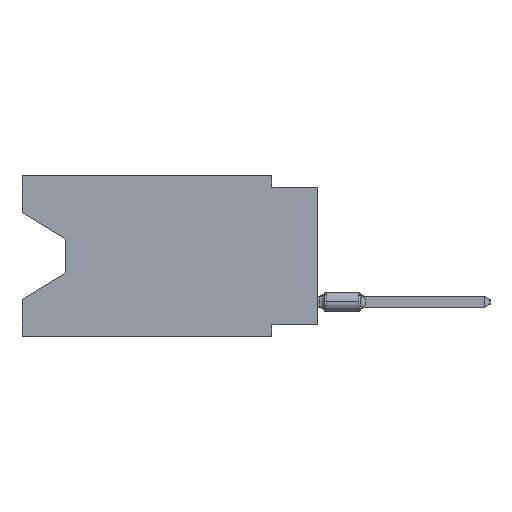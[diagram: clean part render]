
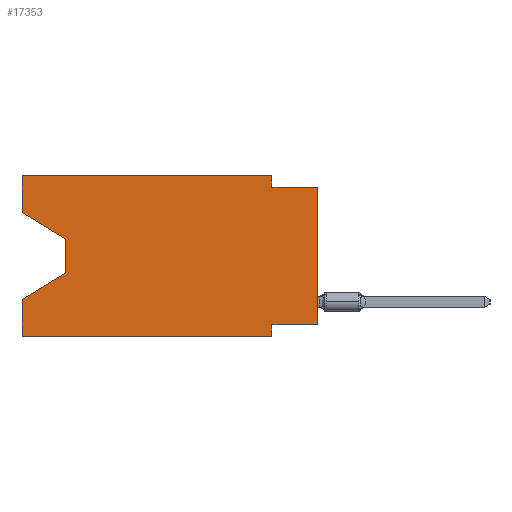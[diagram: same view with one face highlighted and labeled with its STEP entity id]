
A CAD part, left-side view. The second image highlights one B-rep face of the part: STEP entity #17353.
In plain terms, the highlighted planar face has unit normal (-1, 0, 0).
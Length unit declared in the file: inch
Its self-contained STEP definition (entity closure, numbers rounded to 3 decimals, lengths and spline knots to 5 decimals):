
#258 = VECTOR ( 'NONE', #22135, 39.37008 ) ;
#825 = VECTOR ( 'NONE', #10488, 39.37008 ) ;
#1271 = DIRECTION ( 'NONE',  ( 0., 0., -1. ) ) ;
#1423 = EDGE_CURVE ( 'NONE', #21118, #28606, #21655, .T. ) ;
#1750 = VECTOR ( 'NONE', #11403, 39.37008 ) ;
#1928 = ORIENTED_EDGE ( 'NONE', *, *, #2291, .F. ) ;
#2100 = CARTESIAN_POINT ( 'NONE',  ( 0., 0.1, 0. ) ) ;
#2234 = CARTESIAN_POINT ( 'NONE',  ( 0., 0., -0.025 ) ) ;
#2291 = EDGE_CURVE ( 'NONE', #29216, #25674, #48464, .T. ) ;
#3452 = EDGE_CURVE ( 'NONE', #37758, #32745, #3753, .T. ) ;
#3753 = LINE ( 'NONE', #53028, #10088 ) ;
#3994 = ORIENTED_EDGE ( 'NONE', *, *, #34579, .T. ) ;
#4494 = EDGE_CURVE ( 'NONE', #48345, #26114, #19072, .T. ) ;
#5089 = VECTOR ( 'NONE', #7130, 39.37008 ) ;
#6282 = DIRECTION ( 'NONE',  ( 1., 0., 0. ) ) ;
#6395 = EDGE_CURVE ( 'NONE', #21118, #26114, #43600, .T. ) ;
#6995 = CARTESIAN_POINT ( 'NONE',  ( 0., 0.645, 0. ) ) ;
#7130 = DIRECTION ( 'NONE',  ( 0., 0.855, -0.519 ) ) ;
#7263 = VECTOR ( 'NONE', #18466, 39.37008 ) ;
#7921 = LINE ( 'NONE', #48055, #54813 ) ;
#8279 = VERTEX_POINT ( 'NONE', #31749 ) ;
#8656 = CARTESIAN_POINT ( 'NONE',  ( 0., 0.645, -0.35 ) ) ;
#9156 = EDGE_LOOP ( 'NONE', ( #3994, #10153, #30671, #20664, #31892, #45302, #55177, #31588, #46629, #54841, #1928, #39590 ) ) ;
#10088 = VECTOR ( 'NONE', #12614, 39.37008 ) ;
#10153 = ORIENTED_EDGE ( 'NONE', *, *, #48498, .T. ) ;
#10488 = DIRECTION ( 'NONE',  ( 0., 0., -1. ) ) ;
#10738 = CARTESIAN_POINT ( 'NONE',  ( 0., 0., -0.025 ) ) ;
#11003 = FACE_OUTER_BOUND ( 'NONE', #9156, .T. ) ;
#11403 = DIRECTION ( 'NONE',  ( 0., -1., 0. ) ) ;
#12052 = DIRECTION ( 'NONE',  ( 0., -0.855, -0.519 ) ) ;
#12614 = DIRECTION ( 'NONE',  ( 0., 1., 0. ) ) ;
#14913 = CARTESIAN_POINT ( 'NONE',  ( 0., 0.645, 0. ) ) ;
#15213 = CARTESIAN_POINT ( 'NONE',  ( 0., 0.55, -0.138 ) ) ;
#16152 = EDGE_CURVE ( 'NONE', #37758, #26342, #22910, .T. ) ;
#16683 = DIRECTION ( 'NONE',  ( 0., 0., -1. ) ) ;
#17353 = ADVANCED_FACE ( 'NONE', ( #11003 ), #28134, .F. ) ;
#18466 = DIRECTION ( 'NONE',  ( 0., 0., 1. ) ) ;
#18622 = VECTOR ( 'NONE', #42407, 39.37008 ) ;
#19072 = LINE ( 'NONE', #27901, #5089 ) ;
#20130 = VERTEX_POINT ( 'NONE', #57515 ) ;
#20664 = ORIENTED_EDGE ( 'NONE', *, *, #6395, .F. ) ;
#21118 = VERTEX_POINT ( 'NONE', #52037 ) ;
#21655 = LINE ( 'NONE', #8656, #47965 ) ;
#22135 = DIRECTION ( 'NONE',  ( 0., 0., 1. ) ) ;
#22910 = LINE ( 'NONE', #54994, #7263 ) ;
#23464 = CARTESIAN_POINT ( 'NONE',  ( 0., 0.645, -0.26975 ) ) ;
#23506 = LINE ( 'NONE', #14913, #258 ) ;
#24939 = CARTESIAN_POINT ( 'NONE',  ( 0., 0.1, -0.35 ) ) ;
#24989 = CARTESIAN_POINT ( 'NONE',  ( 0., 0.1, -0.35 ) ) ;
#25674 = VERTEX_POINT ( 'NONE', #50648 ) ;
#25871 = EDGE_CURVE ( 'NONE', #20130, #26342, #41789, .T. ) ;
#26114 = VERTEX_POINT ( 'NONE', #23464 ) ;
#26342 = VERTEX_POINT ( 'NONE', #10738 ) ;
#26631 = DIRECTION ( 'NONE',  ( 0., -1., 0. ) ) ;
#27229 = DIRECTION ( 'NONE',  ( 0., -1., 0. ) ) ;
#27901 = CARTESIAN_POINT ( 'NONE',  ( 0., 0.55, -0.212 ) ) ;
#28134 = PLANE ( 'NONE',  #46890 ) ;
#28606 = VERTEX_POINT ( 'NONE', #24989 ) ;
#29063 = CARTESIAN_POINT ( 'NONE',  ( 0., 0.55, -0.212 ) ) ;
#29216 = VERTEX_POINT ( 'NONE', #57678 ) ;
#30125 = EDGE_CURVE ( 'NONE', #32745, #28606, #56480, .T. ) ;
#30671 = ORIENTED_EDGE ( 'NONE', *, *, #4494, .T. ) ;
#31147 = EDGE_CURVE ( 'NONE', #25674, #20130, #51982, .T. ) ;
#31588 = ORIENTED_EDGE ( 'NONE', *, *, #16152, .T. ) ;
#31749 = CARTESIAN_POINT ( 'NONE',  ( 0., 0.645, -0.08025 ) ) ;
#31892 = ORIENTED_EDGE ( 'NONE', *, *, #1423, .T. ) ;
#32745 = VERTEX_POINT ( 'NONE', #58253 ) ;
#33817 = VERTEX_POINT ( 'NONE', #15213 ) ;
#34340 = VECTOR ( 'NONE', #26631, 39.37008 ) ;
#34579 = EDGE_CURVE ( 'NONE', #8279, #33817, #7921, .T. ) ;
#37431 = EDGE_CURVE ( 'NONE', #8279, #29216, #23506, .T. ) ;
#37758 = VERTEX_POINT ( 'NONE', #44698 ) ;
#37813 = DIRECTION ( 'NONE',  ( 0., 0., -1. ) ) ;
#38483 = VECTOR ( 'NONE', #16683, 39.37008 ) ;
#39590 = ORIENTED_EDGE ( 'NONE', *, *, #37431, .F. ) ;
#39979 = LINE ( 'NONE', #57978, #38483 ) ;
#41789 = LINE ( 'NONE', #2234, #1750 ) ;
#42407 = DIRECTION ( 'NONE',  ( 0., 0., 1. ) ) ;
#43600 = LINE ( 'NONE', #6995, #18622 ) ;
#44698 = CARTESIAN_POINT ( 'NONE',  ( 0., 0., -0.325 ) ) ;
#45302 = ORIENTED_EDGE ( 'NONE', *, *, #30125, .F. ) ;
#46629 = ORIENTED_EDGE ( 'NONE', *, *, #25871, .F. ) ;
#46890 = AXIS2_PLACEMENT_3D ( 'NONE', #51132, #6282, #1271 ) ;
#47965 = VECTOR ( 'NONE', #27229, 39.37008 ) ;
#48055 = CARTESIAN_POINT ( 'NONE',  ( 0., 0.645, -0.08025 ) ) ;
#48345 = VERTEX_POINT ( 'NONE', #29063 ) ;
#48464 = LINE ( 'NONE', #57900, #34340 ) ;
#48498 = EDGE_CURVE ( 'NONE', #33817, #48345, #39979, .T. ) ;
#50648 = CARTESIAN_POINT ( 'NONE',  ( 0., 0.1, 0. ) ) ;
#51132 = CARTESIAN_POINT ( 'NONE',  ( 0., 0.645, 0. ) ) ;
#51982 = LINE ( 'NONE', #2100, #56500 ) ;
#52037 = CARTESIAN_POINT ( 'NONE',  ( 0., 0.645, -0.35 ) ) ;
#53028 = CARTESIAN_POINT ( 'NONE',  ( 0., 0., -0.325 ) ) ;
#54813 = VECTOR ( 'NONE', #12052, 39.37008 ) ;
#54841 = ORIENTED_EDGE ( 'NONE', *, *, #31147, .F. ) ;
#54994 = CARTESIAN_POINT ( 'NONE',  ( 0., 0., 0. ) ) ;
#55177 = ORIENTED_EDGE ( 'NONE', *, *, #3452, .F. ) ;
#56480 = LINE ( 'NONE', #24939, #825 ) ;
#56500 = VECTOR ( 'NONE', #37813, 39.37008 ) ;
#57515 = CARTESIAN_POINT ( 'NONE',  ( 0., 0.1, -0.025 ) ) ;
#57678 = CARTESIAN_POINT ( 'NONE',  ( 0., 0.645, 0. ) ) ;
#57900 = CARTESIAN_POINT ( 'NONE',  ( 0., 0.645, 0. ) ) ;
#57978 = CARTESIAN_POINT ( 'NONE',  ( 0., 0.55, -0.138 ) ) ;
#58253 = CARTESIAN_POINT ( 'NONE',  ( 0., 0.1, -0.325 ) ) ;
